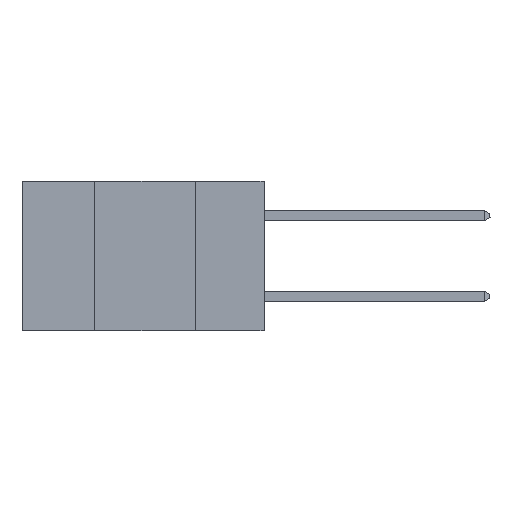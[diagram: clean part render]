
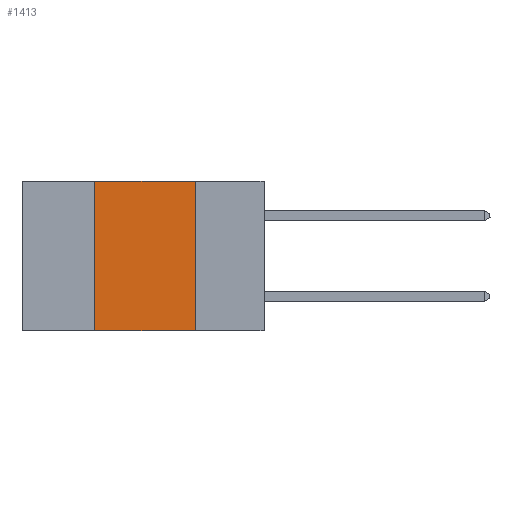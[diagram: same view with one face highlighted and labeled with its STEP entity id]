
A CAD part, left-side view. The second image highlights one B-rep face of the part: STEP entity #1413.
In plain terms, the highlighted planar face has unit normal (-1, 0, 0).
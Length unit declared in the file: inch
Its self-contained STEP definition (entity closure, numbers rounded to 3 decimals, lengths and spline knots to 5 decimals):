
#1413 = ADVANCED_FACE ( 'NONE', ( #15404 ), #11823, .F. ) ;
#4283 = VERTEX_POINT ( 'NONE', #25547 ) ;
#4284 = VECTOR ( 'NONE', #31624, 39.37008 ) ;
#5981 = DIRECTION ( 'NONE',  ( 0., 0., -1. ) ) ;
#6380 = ORIENTED_EDGE ( 'NONE', *, *, #31101, .T. ) ;
#8322 = CARTESIAN_POINT ( 'NONE',  ( 0., 0.6, 0. ) ) ;
#9347 = CARTESIAN_POINT ( 'NONE',  ( 0., 0.6, 0. ) ) ;
#9494 = CARTESIAN_POINT ( 'NONE',  ( 0., 0.42, 0. ) ) ;
#9504 = VECTOR ( 'NONE', #25519, 39.37008 ) ;
#11326 = VECTOR ( 'NONE', #27138, 39.37008 ) ;
#11688 = VERTEX_POINT ( 'NONE', #23100 ) ;
#11823 = PLANE ( 'NONE',  #23492 ) ;
#12305 = ORIENTED_EDGE ( 'NONE', *, *, #25033, .F. ) ;
#13158 = VECTOR ( 'NONE', #5981, 39.37008 ) ;
#13609 = CARTESIAN_POINT ( 'NONE',  ( 0., 0.17, 0. ) ) ;
#14291 = DIRECTION ( 'NONE',  ( 1., 0., 0. ) ) ;
#14973 = EDGE_CURVE ( 'NONE', #31389, #11688, #18169, .T. ) ;
#15404 = FACE_OUTER_BOUND ( 'NONE', #20701, .T. ) ;
#18169 = LINE ( 'NONE', #13609, #13158 ) ;
#20433 = VERTEX_POINT ( 'NONE', #22490 ) ;
#20701 = EDGE_LOOP ( 'NONE', ( #27487, #21864, #12305, #6380 ) ) ;
#21144 = DIRECTION ( 'NONE',  ( 0., 0., -1. ) ) ;
#21864 = ORIENTED_EDGE ( 'NONE', *, *, #29151, .F. ) ;
#22490 = CARTESIAN_POINT ( 'NONE',  ( 0., 0.42, 0. ) ) ;
#23045 = CARTESIAN_POINT ( 'NONE',  ( 0., 0.17, 0. ) ) ;
#23100 = CARTESIAN_POINT ( 'NONE',  ( 0., 0.17, -0.37 ) ) ;
#23492 = AXIS2_PLACEMENT_3D ( 'NONE', #9347, #14291, #21144 ) ;
#24148 = LINE ( 'NONE', #8322, #9504 ) ;
#24785 = LINE ( 'NONE', #9494, #11326 ) ;
#25033 = EDGE_CURVE ( 'NONE', #4283, #20433, #24785, .T. ) ;
#25519 = DIRECTION ( 'NONE',  ( 0., -1., 0. ) ) ;
#25547 = CARTESIAN_POINT ( 'NONE',  ( 0., 0.42, -0.37 ) ) ;
#26247 = LINE ( 'NONE', #31931, #4284 ) ;
#27138 = DIRECTION ( 'NONE',  ( 0., 0., 1. ) ) ;
#27487 = ORIENTED_EDGE ( 'NONE', *, *, #14973, .F. ) ;
#29151 = EDGE_CURVE ( 'NONE', #20433, #31389, #24148, .T. ) ;
#31101 = EDGE_CURVE ( 'NONE', #4283, #11688, #26247, .T. ) ;
#31389 = VERTEX_POINT ( 'NONE', #23045 ) ;
#31624 = DIRECTION ( 'NONE',  ( 0., -1., 0. ) ) ;
#31931 = CARTESIAN_POINT ( 'NONE',  ( 0., 0.6, -0.37 ) ) ;
